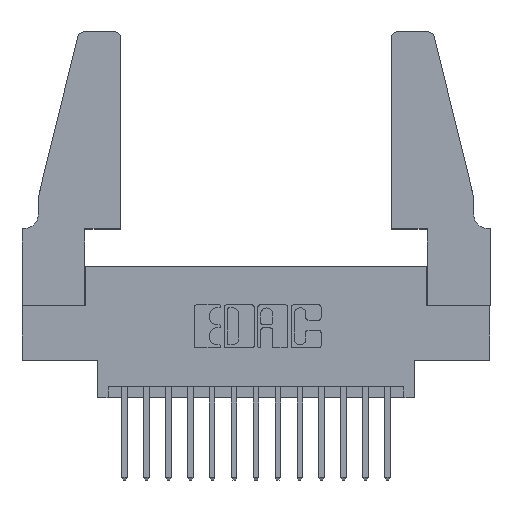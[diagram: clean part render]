
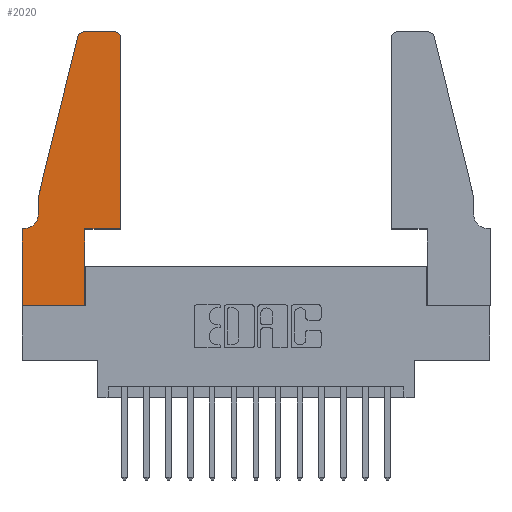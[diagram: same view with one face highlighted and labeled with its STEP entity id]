
A CAD part, top view. The second image highlights one B-rep face of the part: STEP entity #2020.
In plain terms, the highlighted planar face has unit normal (0, 0, 1).
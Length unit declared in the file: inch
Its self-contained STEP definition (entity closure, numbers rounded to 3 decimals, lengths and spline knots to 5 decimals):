
#122 = VECTOR ( 'NONE', #14065, 39.37008 ) ;
#180 = VECTOR ( 'NONE', #15259, 39.37008 ) ;
#407 = CARTESIAN_POINT ( 'NONE',  ( 0.25487, 1.22718, 0.37 ) ) ;
#597 = CIRCLE ( 'NONE', #4334, 0.07 ) ;
#616 = CARTESIAN_POINT ( 'NONE',  ( 0.4505, 0.35, 0.37 ) ) ;
#655 = EDGE_CURVE ( 'NONE', #2836, #14074, #11253, .T. ) ;
#683 = VERTEX_POINT ( 'NONE', #2361 ) ;
#828 = VERTEX_POINT ( 'NONE', #13121 ) ;
#853 = CARTESIAN_POINT ( 'NONE',  ( 0., 0., 0.37 ) ) ;
#863 = VERTEX_POINT ( 'NONE', #12995 ) ;
#1053 = DIRECTION ( 'NONE',  ( 0., 1., 0. ) ) ;
#1095 = VERTEX_POINT ( 'NONE', #407 ) ;
#1235 = PLANE ( 'NONE',  #7376 ) ;
#1388 = CARTESIAN_POINT ( 'NONE',  ( 0.284, 1.25, 0.37 ) ) ;
#1664 = CARTESIAN_POINT ( 'NONE',  ( 0.0055, 0.35, 0.37 ) ) ;
#1696 = CARTESIAN_POINT ( 'NONE',  ( 0., 0., 0.37 ) ) ;
#2020 = ADVANCED_FACE ( 'NONE', ( #14008 ), #1235, .T. ) ;
#2151 = VERTEX_POINT ( 'NONE', #13216 ) ;
#2361 = CARTESIAN_POINT ( 'NONE',  ( 0.0755, 0.42, 0.37 ) ) ;
#2598 = LINE ( 'NONE', #15578, #15880 ) ;
#2636 = DIRECTION ( 'NONE',  ( 1., 0., 0. ) ) ;
#2688 = VECTOR ( 'NONE', #14439, 39.37008 ) ;
#2836 = VERTEX_POINT ( 'NONE', #11301 ) ;
#2914 = EDGE_CURVE ( 'NONE', #5559, #1095, #8434, .T. ) ;
#3023 = EDGE_CURVE ( 'NONE', #6652, #2836, #9660, .T. ) ;
#3102 = DIRECTION ( 'NONE',  ( 0., -1., 0. ) ) ;
#3343 = CARTESIAN_POINT ( 'NONE',  ( 0.2865, 0.35, 0.37 ) ) ;
#3833 = CARTESIAN_POINT ( 'NONE',  ( 0., 0.35, 0.37 ) ) ;
#3984 = EDGE_CURVE ( 'NONE', #6830, #828, #9018, .T. ) ;
#4226 = ORIENTED_EDGE ( 'NONE', *, *, #6083, .T. ) ;
#4334 = AXIS2_PLACEMENT_3D ( 'NONE', #9536, #5724, #15917 ) ;
#5038 = EDGE_LOOP ( 'NONE', ( #13679, #13956, #8969, #4226, #8733, #14540, #13440, #7930, #13901, #7921, #15708, #11396 ) ) ;
#5427 = DIRECTION ( 'NONE',  ( 1., 0., 0. ) ) ;
#5488 = LINE ( 'NONE', #15061, #9044 ) ;
#5549 = DIRECTION ( 'NONE',  ( 1., 0., 0. ) ) ;
#5559 = VERTEX_POINT ( 'NONE', #1388 ) ;
#5724 = DIRECTION ( 'NONE',  ( 0., 0., -1. ) ) ;
#6083 = EDGE_CURVE ( 'NONE', #11836, #683, #15305, .T. ) ;
#6329 = EDGE_CURVE ( 'NONE', #683, #6652, #597, .T. ) ;
#6469 = AXIS2_PLACEMENT_3D ( 'NONE', #15594, #13274, #5549 ) ;
#6555 = LINE ( 'NONE', #9507, #15687 ) ;
#6557 = CARTESIAN_POINT ( 'NONE',  ( 0.0755, 0.5, 0.37 ) ) ;
#6649 = EDGE_CURVE ( 'NONE', #14074, #9516, #2598, .T. ) ;
#6652 = VERTEX_POINT ( 'NONE', #1664 ) ;
#6830 = VERTEX_POINT ( 'NONE', #3343 ) ;
#6888 = DIRECTION ( 'NONE',  ( -1., 0., 0. ) ) ;
#7098 = LINE ( 'NONE', #9980, #14272 ) ;
#7130 = EDGE_CURVE ( 'NONE', #9516, #6830, #7098, .T. ) ;
#7136 = DIRECTION ( 'NONE',  ( 1., 0., 0. ) ) ;
#7198 = EDGE_CURVE ( 'NONE', #1095, #11836, #13457, .T. ) ;
#7376 = AXIS2_PLACEMENT_3D ( 'NONE', #3833, #8933, #2636 ) ;
#7921 = ORIENTED_EDGE ( 'NONE', *, *, #3984, .T. ) ;
#7930 = ORIENTED_EDGE ( 'NONE', *, *, #6649, .T. ) ;
#7998 = CARTESIAN_POINT ( 'NONE',  ( 0.2865, 0., 0.37 ) ) ;
#8434 = CIRCLE ( 'NONE', #6469, 0.03 ) ;
#8733 = ORIENTED_EDGE ( 'NONE', *, *, #6329, .T. ) ;
#8933 = DIRECTION ( 'NONE',  ( 0., 0., 1. ) ) ;
#8969 = ORIENTED_EDGE ( 'NONE', *, *, #7198, .T. ) ;
#9018 = LINE ( 'NONE', #616, #2688 ) ;
#9044 = VECTOR ( 'NONE', #11086, 39.37008 ) ;
#9213 = CARTESIAN_POINT ( 'NONE',  ( 0.0755, 0.35, 0.37 ) ) ;
#9507 = CARTESIAN_POINT ( 'NONE',  ( 0.2605, 1.25, 0.37 ) ) ;
#9516 = VERTEX_POINT ( 'NONE', #7998 ) ;
#9536 = CARTESIAN_POINT ( 'NONE',  ( 0.0055, 0.42, 0.37 ) ) ;
#9660 = LINE ( 'NONE', #9213, #122 ) ;
#9980 = CARTESIAN_POINT ( 'NONE',  ( 0.2865, 0.35, 0.37 ) ) ;
#10140 = CARTESIAN_POINT ( 'NONE',  ( 0.0755, 0.5, 0.37 ) ) ;
#10250 = AXIS2_PLACEMENT_3D ( 'NONE', #14595, #13402, #7136 ) ;
#11086 = DIRECTION ( 'NONE',  ( 0., 1., 0. ) ) ;
#11253 = LINE ( 'NONE', #1696, #14248 ) ;
#11301 = CARTESIAN_POINT ( 'NONE',  ( 0., 0.35, 0.37 ) ) ;
#11302 = CARTESIAN_POINT ( 'NONE',  ( 0.0755, 0.5, 0.37 ) ) ;
#11396 = ORIENTED_EDGE ( 'NONE', *, *, #15137, .T. ) ;
#11836 = VERTEX_POINT ( 'NONE', #11302 ) ;
#12465 = EDGE_CURVE ( 'NONE', #828, #863, #5488, .T. ) ;
#12995 = CARTESIAN_POINT ( 'NONE',  ( 0.4505, 1.22, 0.37 ) ) ;
#13121 = CARTESIAN_POINT ( 'NONE',  ( 0.4505, 0.35, 0.37 ) ) ;
#13216 = CARTESIAN_POINT ( 'NONE',  ( 0.4205, 1.25, 0.37 ) ) ;
#13274 = DIRECTION ( 'NONE',  ( 0., 0., 1. ) ) ;
#13402 = DIRECTION ( 'NONE',  ( 0., 0., 1. ) ) ;
#13440 = ORIENTED_EDGE ( 'NONE', *, *, #655, .T. ) ;
#13457 = LINE ( 'NONE', #10140, #180 ) ;
#13679 = ORIENTED_EDGE ( 'NONE', *, *, #16367, .T. ) ;
#13901 = ORIENTED_EDGE ( 'NONE', *, *, #7130, .T. ) ;
#13956 = ORIENTED_EDGE ( 'NONE', *, *, #2914, .T. ) ;
#14008 = FACE_OUTER_BOUND ( 'NONE', #5038, .T. ) ;
#14065 = DIRECTION ( 'NONE',  ( -1., 0., 0. ) ) ;
#14074 = VERTEX_POINT ( 'NONE', #853 ) ;
#14248 = VECTOR ( 'NONE', #3102, 39.37008 ) ;
#14272 = VECTOR ( 'NONE', #1053, 39.37008 ) ;
#14439 = DIRECTION ( 'NONE',  ( 1., 0., 0. ) ) ;
#14540 = ORIENTED_EDGE ( 'NONE', *, *, #3023, .T. ) ;
#14595 = CARTESIAN_POINT ( 'NONE',  ( 0.4205, 1.22, 0.37 ) ) ;
#14705 = VECTOR ( 'NONE', #15212, 39.37008 ) ;
#15061 = CARTESIAN_POINT ( 'NONE',  ( 0.4505, 0.35, 0.37 ) ) ;
#15137 = EDGE_CURVE ( 'NONE', #863, #2151, #15346, .T. ) ;
#15212 = DIRECTION ( 'NONE',  ( 0., -1., 0. ) ) ;
#15259 = DIRECTION ( 'NONE',  ( -0.239, -0.971, 0. ) ) ;
#15305 = LINE ( 'NONE', #6557, #14705 ) ;
#15346 = CIRCLE ( 'NONE', #10250, 0.03 ) ;
#15578 = CARTESIAN_POINT ( 'NONE',  ( 0., 0., 0.37 ) ) ;
#15594 = CARTESIAN_POINT ( 'NONE',  ( 0.284, 1.22, 0.37 ) ) ;
#15687 = VECTOR ( 'NONE', #6888, 39.37008 ) ;
#15708 = ORIENTED_EDGE ( 'NONE', *, *, #12465, .T. ) ;
#15880 = VECTOR ( 'NONE', #5427, 39.37008 ) ;
#15917 = DIRECTION ( 'NONE',  ( -1., 0., 0. ) ) ;
#16367 = EDGE_CURVE ( 'NONE', #2151, #5559, #6555, .T. ) ;
